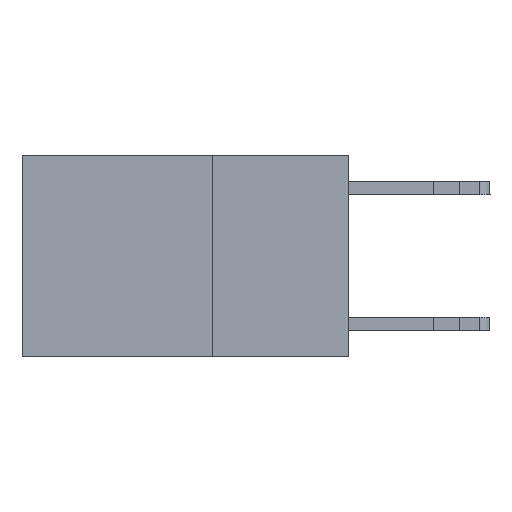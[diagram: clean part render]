
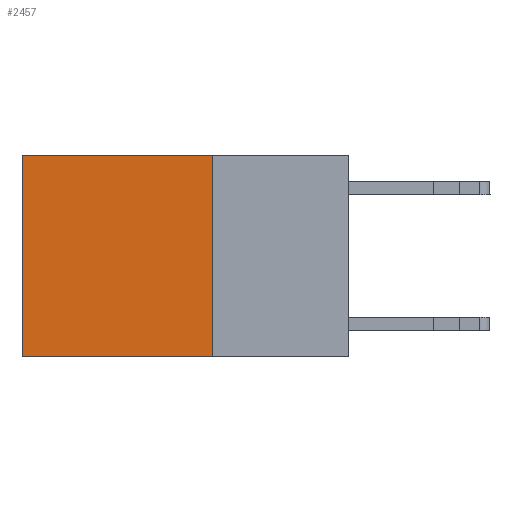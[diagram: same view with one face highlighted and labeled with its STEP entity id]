
A CAD part, left-side view. The second image highlights one B-rep face of the part: STEP entity #2457.
In plain terms, the highlighted planar face has unit normal (-1, 0, 0).
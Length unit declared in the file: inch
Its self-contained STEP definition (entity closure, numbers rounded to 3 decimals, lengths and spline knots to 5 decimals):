
#247 = CARTESIAN_POINT ( 'NONE',  ( 0.2625, 0.25, 0. ) ) ;
#726 = EDGE_CURVE ( 'NONE', #2376, #3871, #8262, .T. ) ;
#820 = CARTESIAN_POINT ( 'NONE',  ( 0.2625, 0.25, 0. ) ) ;
#1330 = CARTESIAN_POINT ( 'NONE',  ( 0.2625, 0.6, 0. ) ) ;
#1379 = CARTESIAN_POINT ( 'NONE',  ( 0.2625, 0.25, 0. ) ) ;
#1628 = DIRECTION ( 'NONE',  ( 0., 0., -1. ) ) ;
#1972 = FACE_OUTER_BOUND ( 'NONE', #6561, .T. ) ;
#2376 = VERTEX_POINT ( 'NONE', #11679 ) ;
#2437 = DIRECTION ( 'NONE',  ( 0., 0., -1. ) ) ;
#2457 = ADVANCED_FACE ( 'NONE', ( #1972 ), #7677, .F. ) ;
#2556 = CARTESIAN_POINT ( 'NONE',  ( 0.2625, 0.25, 0. ) ) ;
#2937 = DIRECTION ( 'NONE',  ( 0., 1., 0. ) ) ;
#3527 = VECTOR ( 'NONE', #2937, 39.37008 ) ;
#3871 = VERTEX_POINT ( 'NONE', #7270 ) ;
#4054 = ORIENTED_EDGE ( 'NONE', *, *, #10849, .T. ) ;
#4217 = EDGE_CURVE ( 'NONE', #6643, #2376, #5052, .T. ) ;
#4730 = CARTESIAN_POINT ( 'NONE',  ( 0.2625, 0.25, -0.37 ) ) ;
#5052 = LINE ( 'NONE', #2556, #7521 ) ;
#6478 = ORIENTED_EDGE ( 'NONE', *, *, #4217, .F. ) ;
#6555 = AXIS2_PLACEMENT_3D ( 'NONE', #1379, #8729, #2437 ) ;
#6561 = EDGE_LOOP ( 'NONE', ( #4054, #13498, #6478, #12021 ) ) ;
#6643 = VERTEX_POINT ( 'NONE', #247 ) ;
#6862 = CARTESIAN_POINT ( 'NONE',  ( 0.2625, 0.6, 0. ) ) ;
#7259 = LINE ( 'NONE', #6862, #12766 ) ;
#7270 = CARTESIAN_POINT ( 'NONE',  ( 0.2625, 0.6, -0.37 ) ) ;
#7521 = VECTOR ( 'NONE', #11965, 39.37008 ) ;
#7630 = LINE ( 'NONE', #820, #3527 ) ;
#7677 = PLANE ( 'NONE',  #6555 ) ;
#8005 = VERTEX_POINT ( 'NONE', #1330 ) ;
#8262 = LINE ( 'NONE', #4730, #13417 ) ;
#8358 = EDGE_CURVE ( 'NONE', #6643, #8005, #7630, .T. ) ;
#8729 = DIRECTION ( 'NONE',  ( 1., 0., 0. ) ) ;
#8823 = DIRECTION ( 'NONE',  ( 0., 1., 0. ) ) ;
#10849 = EDGE_CURVE ( 'NONE', #8005, #3871, #7259, .T. ) ;
#11679 = CARTESIAN_POINT ( 'NONE',  ( 0.2625, 0.25, -0.37 ) ) ;
#11965 = DIRECTION ( 'NONE',  ( 0., 0., -1. ) ) ;
#12021 = ORIENTED_EDGE ( 'NONE', *, *, #8358, .T. ) ;
#12766 = VECTOR ( 'NONE', #1628, 39.37008 ) ;
#13417 = VECTOR ( 'NONE', #8823, 39.37008 ) ;
#13498 = ORIENTED_EDGE ( 'NONE', *, *, #726, .F. ) ;
